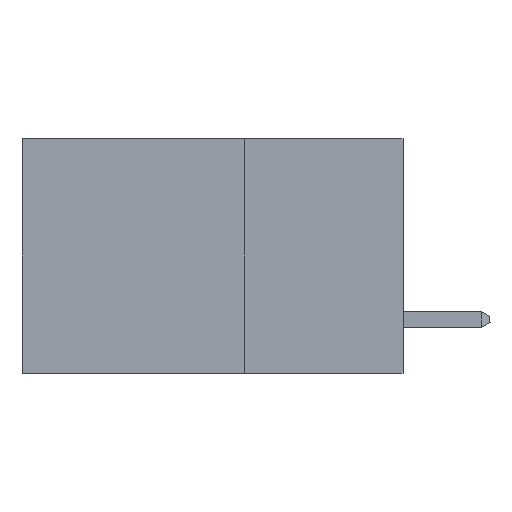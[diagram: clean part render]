
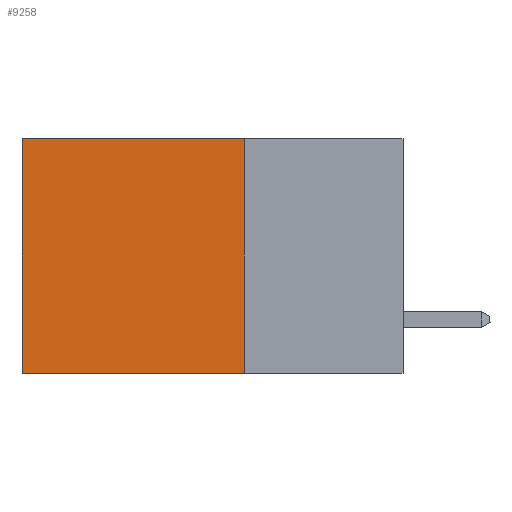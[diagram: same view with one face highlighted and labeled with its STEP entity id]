
A CAD part, left-side view. The second image highlights one B-rep face of the part: STEP entity #9258.
In plain terms, the highlighted planar face has unit normal (-1, 0, 0).
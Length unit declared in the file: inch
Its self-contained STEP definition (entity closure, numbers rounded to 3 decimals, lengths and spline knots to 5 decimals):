
#1054 = FACE_OUTER_BOUND ( 'NONE', #8014, .T. ) ;
#1587 = ORIENTED_EDGE ( 'NONE', *, *, #8220, .F. ) ;
#1890 = DIRECTION ( 'NONE',  ( 1., 0., 0. ) ) ;
#1986 = CARTESIAN_POINT ( 'NONE',  ( 0.2875, 0.25, 0. ) ) ;
#2475 = DIRECTION ( 'NONE',  ( 0., 1., 0. ) ) ;
#3228 = CARTESIAN_POINT ( 'NONE',  ( 0.2875, 0.6, 0. ) ) ;
#3515 = VECTOR ( 'NONE', #5393, 39.37008 ) ;
#3715 = VERTEX_POINT ( 'NONE', #3228 ) ;
#3810 = VECTOR ( 'NONE', #6638, 39.37008 ) ;
#3847 = LINE ( 'NONE', #7270, #4390 ) ;
#4108 = ORIENTED_EDGE ( 'NONE', *, *, #10597, .T. ) ;
#4125 = EDGE_CURVE ( 'NONE', #7875, #5135, #9989, .T. ) ;
#4390 = VECTOR ( 'NONE', #8114, 39.37008 ) ;
#5135 = VERTEX_POINT ( 'NONE', #8054 ) ;
#5193 = VERTEX_POINT ( 'NONE', #7996 ) ;
#5393 = DIRECTION ( 'NONE',  ( 0., 1., 0. ) ) ;
#6371 = CARTESIAN_POINT ( 'NONE',  ( 0.2875, 0.25, 0. ) ) ;
#6638 = DIRECTION ( 'NONE',  ( 0., 0., -1. ) ) ;
#6684 = LINE ( 'NONE', #10081, #7780 ) ;
#7270 = CARTESIAN_POINT ( 'NONE',  ( 0.2875, 0.6, 0. ) ) ;
#7780 = VECTOR ( 'NONE', #2475, 39.37008 ) ;
#7875 = VERTEX_POINT ( 'NONE', #10104 ) ;
#7996 = CARTESIAN_POINT ( 'NONE',  ( 0.2875, 0.6, -0.37 ) ) ;
#8014 = EDGE_LOOP ( 'NONE', ( #10713, #1587, #8158, #4108 ) ) ;
#8054 = CARTESIAN_POINT ( 'NONE',  ( 0.2875, 0.25, -0.37 ) ) ;
#8061 = DIRECTION ( 'NONE',  ( 0., 0., -1. ) ) ;
#8114 = DIRECTION ( 'NONE',  ( 0., 0., -1. ) ) ;
#8158 = ORIENTED_EDGE ( 'NONE', *, *, #4125, .F. ) ;
#8161 = AXIS2_PLACEMENT_3D ( 'NONE', #6371, #1890, #8061 ) ;
#8220 = EDGE_CURVE ( 'NONE', #5135, #5193, #6684, .T. ) ;
#8778 = PLANE ( 'NONE',  #8161 ) ;
#9258 = ADVANCED_FACE ( 'NONE', ( #1054 ), #8778, .F. ) ;
#9441 = EDGE_CURVE ( 'NONE', #3715, #5193, #3847, .T. ) ;
#9936 = CARTESIAN_POINT ( 'NONE',  ( 0.2875, 0.25, 0. ) ) ;
#9989 = LINE ( 'NONE', #9936, #3810 ) ;
#10081 = CARTESIAN_POINT ( 'NONE',  ( 0.2875, 0.25, -0.37 ) ) ;
#10104 = CARTESIAN_POINT ( 'NONE',  ( 0.2875, 0.25, 0. ) ) ;
#10597 = EDGE_CURVE ( 'NONE', #7875, #3715, #10603, .T. ) ;
#10603 = LINE ( 'NONE', #1986, #3515 ) ;
#10713 = ORIENTED_EDGE ( 'NONE', *, *, #9441, .T. ) ;
